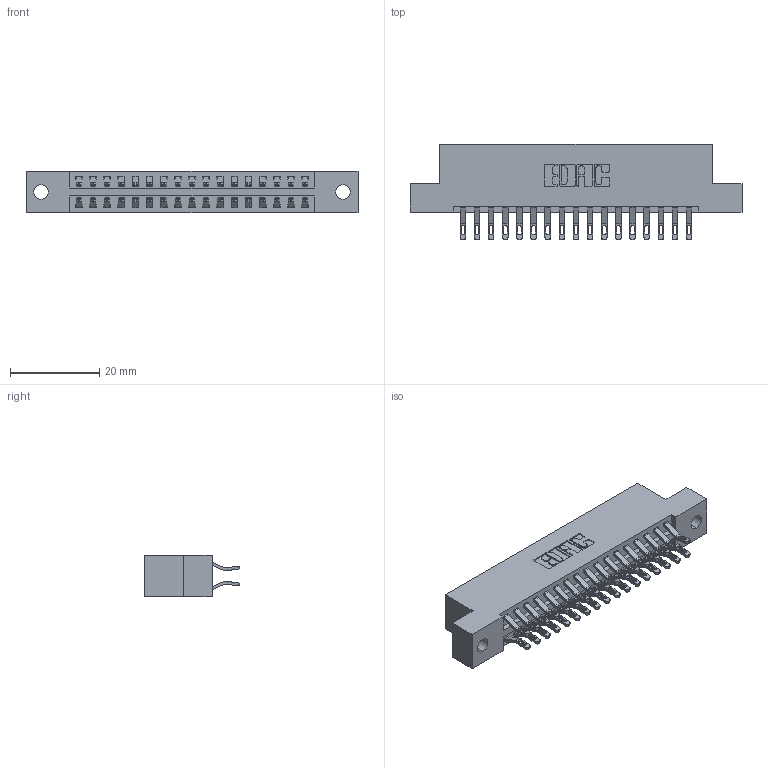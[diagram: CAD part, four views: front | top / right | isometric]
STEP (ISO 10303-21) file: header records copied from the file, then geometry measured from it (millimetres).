
FILE_DESCRIPTION (( 'STEP AP203' ), '1' );
FILE_NAME ('396-034-555-202.STEP', '2018-09-06T01:14:35', ( '' ), ( '' ), 'SwSTEP 2.0', 'SolidWorks 2016', '' );
FILE_SCHEMA (( 'CONFIG_CONTROL_DESIGN' ));
Length unit declared in the file: inch
Products named in the file (3): 345-292-001_555 Tail; 396-034-555-202; 346 Part_Flush Mounting Lugs - 0.128 Dia
Assembly tree (35 placements, depth 2):
  396-034-555-202
    346 Part_Flush Mounting Lugs - 0.128 Dia
    345-292-001_555 Tail  x34
Bounding box: 74.55 x 21.46 x 9.4 mm (x, y, z)
Volume: 7137.2 mm3; surface area: 9499.9 mm2
Topology: 35 solids, 35 shells, 2094 faces, 6551 edges, 4366 vertices
Faces by surface type: plane 1198, cylinder 896
Entity records: 14789 total; most frequent: CARTESIAN_POINT 2506, ORIENTED_EDGE 2410, DIRECTION 2229, EDGE_CURVE 1205, VECTOR 985, LINE 985, VERTEX_POINT 802, AXIS2_PLACEMENT_3D 622
